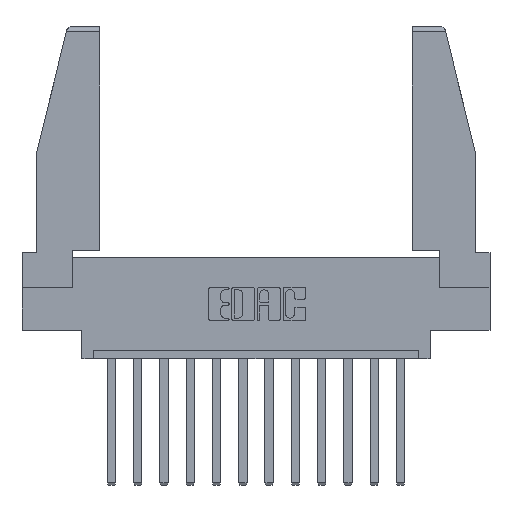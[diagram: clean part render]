
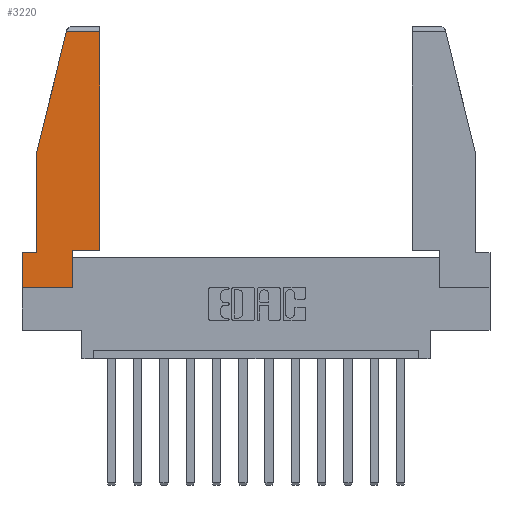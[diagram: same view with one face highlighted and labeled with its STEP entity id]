
A CAD part, top view. The second image highlights one B-rep face of the part: STEP entity #3220.
In plain terms, the highlighted planar face has unit normal (0, 0, 1).
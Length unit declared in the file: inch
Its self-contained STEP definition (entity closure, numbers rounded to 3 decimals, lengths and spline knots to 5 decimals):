
#42 = EDGE_CURVE ( 'NONE', #13692, #11817, #6305, .T. ) ;
#100 = VECTOR ( 'NONE', #6354, 39.37008 ) ;
#385 = CARTESIAN_POINT ( 'NONE',  ( 0., 0., 0. ) ) ;
#485 = CARTESIAN_POINT ( 'NONE',  ( 0.297, 0., 0. ) ) ;
#507 = VERTEX_POINT ( 'NONE', #6288 ) ;
#684 = CARTESIAN_POINT ( 'NONE',  ( 0.271, 1.55, 0. ) ) ;
#1060 = CARTESIAN_POINT ( 'NONE',  ( 0., 0., 0. ) ) ;
#1358 = EDGE_LOOP ( 'NONE', ( #4261, #2612, #10605, #6127, #11798, #9385, #10328, #13198, #2571 ) ) ;
#1485 = EDGE_CURVE ( 'NONE', #11817, #5968, #2280, .T. ) ;
#1687 = DIRECTION ( 'NONE',  ( 1., 0., 0. ) ) ;
#1748 = DIRECTION ( 'NONE',  ( 1., 0., 0. ) ) ;
#2216 = PLANE ( 'NONE',  #14158 ) ;
#2280 = LINE ( 'NONE', #10303, #13097 ) ;
#2571 = ORIENTED_EDGE ( 'NONE', *, *, #7857, .T. ) ;
#2612 = ORIENTED_EDGE ( 'NONE', *, *, #4680, .T. ) ;
#2996 = VECTOR ( 'NONE', #10949, 39.37008 ) ;
#3038 = LINE ( 'NONE', #9095, #3770 ) ;
#3220 = ADVANCED_FACE ( 'NONE', ( #8585 ), #2216, .T. ) ;
#3309 = VECTOR ( 'NONE', #1748, 39.37008 ) ;
#3693 = CARTESIAN_POINT ( 'NONE',  ( 0.461, 1.52, 0. ) ) ;
#3770 = VECTOR ( 'NONE', #11481, 39.37008 ) ;
#4052 = CARTESIAN_POINT ( 'NONE',  ( 0.297, 0.223, 0. ) ) ;
#4261 = ORIENTED_EDGE ( 'NONE', *, *, #6091, .T. ) ;
#4666 = DIRECTION ( 'NONE',  ( 1., 0., 0. ) ) ;
#4680 = EDGE_CURVE ( 'NONE', #5986, #13692, #3038, .T. ) ;
#4696 = VERTEX_POINT ( 'NONE', #5779 ) ;
#4708 = CARTESIAN_POINT ( 'NONE',  ( 0.2636, 1.52, 0. ) ) ;
#4892 = VECTOR ( 'NONE', #6109, 39.37008 ) ;
#5077 = CARTESIAN_POINT ( 'NONE',  ( 0.086, 0.8, 0. ) ) ;
#5081 = VERTEX_POINT ( 'NONE', #11104 ) ;
#5411 = LINE ( 'NONE', #9683, #4892 ) ;
#5527 = CARTESIAN_POINT ( 'NONE',  ( 0., 0.21, 0. ) ) ;
#5779 = CARTESIAN_POINT ( 'NONE',  ( 0., 0.21, 0. ) ) ;
#5968 = VERTEX_POINT ( 'NONE', #11890 ) ;
#5986 = VERTEX_POINT ( 'NONE', #3693 ) ;
#6091 = EDGE_CURVE ( 'NONE', #6424, #5986, #10500, .T. ) ;
#6109 = DIRECTION ( 'NONE',  ( 0., -1., 0. ) ) ;
#6127 = ORIENTED_EDGE ( 'NONE', *, *, #1485, .T. ) ;
#6288 = CARTESIAN_POINT ( 'NONE',  ( 0.297, 0.223, 0. ) ) ;
#6305 = LINE ( 'NONE', #684, #100 ) ;
#6354 = DIRECTION ( 'NONE',  ( -0.239, -0.971, 0. ) ) ;
#6424 = VERTEX_POINT ( 'NONE', #7671 ) ;
#7218 = LINE ( 'NONE', #5527, #7767 ) ;
#7671 = CARTESIAN_POINT ( 'NONE',  ( 0.461, 0.223, 0. ) ) ;
#7767 = VECTOR ( 'NONE', #11281, 39.37008 ) ;
#7813 = LINE ( 'NONE', #14499, #12600 ) ;
#7857 = EDGE_CURVE ( 'NONE', #507, #6424, #14482, .T. ) ;
#8585 = FACE_OUTER_BOUND ( 'NONE', #1358, .T. ) ;
#9002 = EDGE_CURVE ( 'NONE', #11338, #5081, #7813, .T. ) ;
#9095 = CARTESIAN_POINT ( 'NONE',  ( 0., 1.52, 0. ) ) ;
#9385 = ORIENTED_EDGE ( 'NONE', *, *, #9480, .T. ) ;
#9480 = EDGE_CURVE ( 'NONE', #4696, #11338, #5411, .T. ) ;
#9683 = CARTESIAN_POINT ( 'NONE',  ( 0., 0.21, 0. ) ) ;
#9772 = CARTESIAN_POINT ( 'NONE',  ( 0.461, 0.223, 0. ) ) ;
#10285 = EDGE_CURVE ( 'NONE', #5968, #4696, #7218, .T. ) ;
#10303 = CARTESIAN_POINT ( 'NONE',  ( 0.086, 0.8, 0. ) ) ;
#10328 = ORIENTED_EDGE ( 'NONE', *, *, #9002, .T. ) ;
#10500 = LINE ( 'NONE', #9772, #2996 ) ;
#10605 = ORIENTED_EDGE ( 'NONE', *, *, #42, .T. ) ;
#10949 = DIRECTION ( 'NONE',  ( 0., 1., 0. ) ) ;
#11067 = VECTOR ( 'NONE', #14337, 39.37008 ) ;
#11104 = CARTESIAN_POINT ( 'NONE',  ( 0.297, 0., 0. ) ) ;
#11281 = DIRECTION ( 'NONE',  ( -1., 0., 0. ) ) ;
#11338 = VERTEX_POINT ( 'NONE', #385 ) ;
#11432 = EDGE_CURVE ( 'NONE', #5081, #507, #14718, .T. ) ;
#11481 = DIRECTION ( 'NONE',  ( -1., 0., 0. ) ) ;
#11798 = ORIENTED_EDGE ( 'NONE', *, *, #10285, .T. ) ;
#11817 = VERTEX_POINT ( 'NONE', #5077 ) ;
#11890 = CARTESIAN_POINT ( 'NONE',  ( 0.086, 0.21, 0. ) ) ;
#12600 = VECTOR ( 'NONE', #1687, 39.37008 ) ;
#13097 = VECTOR ( 'NONE', #13959, 39.37008 ) ;
#13198 = ORIENTED_EDGE ( 'NONE', *, *, #11432, .T. ) ;
#13692 = VERTEX_POINT ( 'NONE', #4708 ) ;
#13956 = DIRECTION ( 'NONE',  ( 0., 0., 1. ) ) ;
#13959 = DIRECTION ( 'NONE',  ( 0., -1., 0. ) ) ;
#14158 = AXIS2_PLACEMENT_3D ( 'NONE', #1060, #13956, #4666 ) ;
#14337 = DIRECTION ( 'NONE',  ( 0., 1., 0. ) ) ;
#14482 = LINE ( 'NONE', #4052, #3309 ) ;
#14499 = CARTESIAN_POINT ( 'NONE',  ( 0., 0., 0. ) ) ;
#14718 = LINE ( 'NONE', #485, #11067 ) ;
